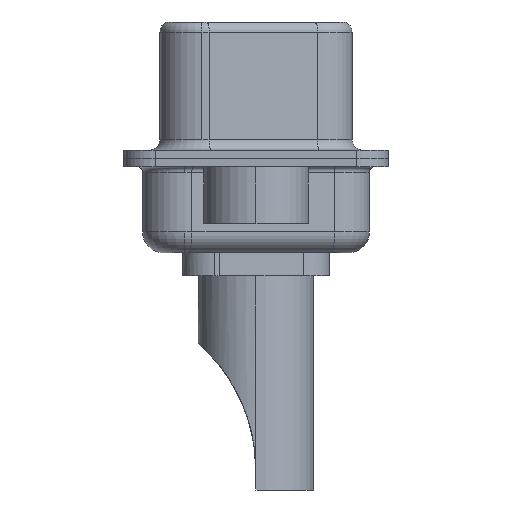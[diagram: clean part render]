
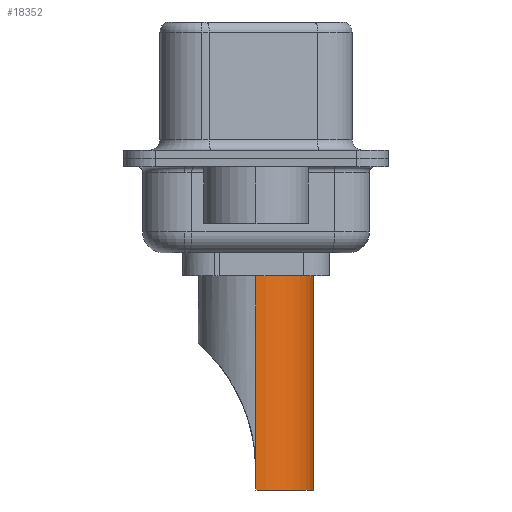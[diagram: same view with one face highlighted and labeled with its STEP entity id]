
A CAD part, left-side view. The second image highlights one B-rep face of the part: STEP entity #18352.
In plain terms, the highlighted cylindrical face has radius 2.75 mm (diameter 5.5 mm), a partial arc.
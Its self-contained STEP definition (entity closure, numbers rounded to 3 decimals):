
#19 = CARTESIAN_POINT ( 'NONE',  ( -2.75, 0., 4.234 ) ) ;
#313 = VECTOR ( 'NONE', #6127, 1000. ) ;
#859 = EDGE_CURVE ( 'NONE', #14765, #18203, #14205, .T. ) ;
#2672 = EDGE_LOOP ( 'NONE', ( #3869, #10466, #15259, #14167, #17523, #11882 ) ) ;
#2728 = CARTESIAN_POINT ( 'NONE',  ( -2.75, 0., -8.7 ) ) ;
#3127 = DIRECTION ( 'NONE',  ( 0., 0., 1. ) ) ;
#3869 = ORIENTED_EDGE ( 'NONE', *, *, #8987, .F. ) ;
#4400 = CIRCLE ( 'NONE', #14729, 2.75 ) ;
#5070 = AXIS2_PLACEMENT_3D ( 'NONE', #7988, #18836, #9633 ) ;
#5502 = VECTOR ( 'NONE', #15358, 1000. ) ;
#5547 = CARTESIAN_POINT ( 'NONE',  ( 2.75, 0., 1.5 ) ) ;
#5851 = CARTESIAN_POINT ( 'NONE',  ( 2.75, 0., 4.234 ) ) ;
#5928 = FACE_OUTER_BOUND ( 'NONE', #2672, .T. ) ;
#6127 = DIRECTION ( 'NONE',  ( 0., 0., -1. ) ) ;
#6656 = LINE ( 'NONE', #19, #15074 ) ;
#7647 = CARTESIAN_POINT ( 'NONE',  ( -2.75, 0., -8.7 ) ) ;
#7988 = CARTESIAN_POINT ( 'NONE',  ( 0., 0., -8.7 ) ) ;
#7994 = CARTESIAN_POINT ( 'NONE',  ( -2.75, 0., 1.5 ) ) ;
#8199 = LINE ( 'NONE', #7647, #313 ) ;
#8392 = DIRECTION ( 'NONE',  ( 0., 0., -1. ) ) ;
#8915 = EDGE_CURVE ( 'NONE', #16724, #17880, #8199, .T. ) ;
#8987 = EDGE_CURVE ( 'NONE', #16724, #19312, #6656, .T. ) ;
#9453 = VERTEX_POINT ( 'NONE', #5547 ) ;
#9493 = DIRECTION ( 'NONE',  ( 0., 0., 1. ) ) ;
#9633 = DIRECTION ( 'NONE',  ( 1., 0., 0. ) ) ;
#10131 = DIRECTION ( 'NONE',  ( 0., 0., 1. ) ) ;
#10466 = ORIENTED_EDGE ( 'NONE', *, *, #8915, .T. ) ;
#11324 = EDGE_CURVE ( 'NONE', #19312, #9453, #4400, .T. ) ;
#11882 = ORIENTED_EDGE ( 'NONE', *, *, #11324, .F. ) ;
#11993 = EDGE_CURVE ( 'NONE', #17880, #18203, #18045, .T. ) ;
#12673 = CARTESIAN_POINT ( 'NONE',  ( 0., 0., 1.5 ) ) ;
#13382 = CARTESIAN_POINT ( 'NONE',  ( 2.75, 0., -8.7 ) ) ;
#13949 = LINE ( 'NONE', #5851, #5502 ) ;
#14167 = ORIENTED_EDGE ( 'NONE', *, *, #859, .F. ) ;
#14188 = DIRECTION ( 'NONE',  ( 1., 0., 0. ) ) ;
#14205 = LINE ( 'NONE', #13382, #17719 ) ;
#14729 = AXIS2_PLACEMENT_3D ( 'NONE', #12673, #3127, #14188 ) ;
#14765 = VERTEX_POINT ( 'NONE', #15265 ) ;
#15074 = VECTOR ( 'NONE', #9493, 1000. ) ;
#15259 = ORIENTED_EDGE ( 'NONE', *, *, #11993, .T. ) ;
#15265 = CARTESIAN_POINT ( 'NONE',  ( 2.75, 0., -7.764 ) ) ;
#15358 = DIRECTION ( 'NONE',  ( 0., 0., 1. ) ) ;
#15800 = AXIS2_PLACEMENT_3D ( 'NONE', #16269, #10131, #19321 ) ;
#15940 = CARTESIAN_POINT ( 'NONE',  ( 2.75, 0., -8.7 ) ) ;
#16266 = EDGE_CURVE ( 'NONE', #14765, #9453, #13949, .T. ) ;
#16269 = CARTESIAN_POINT ( 'NONE',  ( 0., 0., 4.234 ) ) ;
#16724 = VERTEX_POINT ( 'NONE', #17004 ) ;
#17004 = CARTESIAN_POINT ( 'NONE',  ( -2.75, 0., -7.764 ) ) ;
#17377 = CYLINDRICAL_SURFACE ( 'NONE', #15800, 2.75 ) ;
#17523 = ORIENTED_EDGE ( 'NONE', *, *, #16266, .T. ) ;
#17719 = VECTOR ( 'NONE', #8392, 1000. ) ;
#17880 = VERTEX_POINT ( 'NONE', #2728 ) ;
#18045 = CIRCLE ( 'NONE', #5070, 2.75 ) ;
#18203 = VERTEX_POINT ( 'NONE', #15940 ) ;
#18352 = ADVANCED_FACE ( 'NONE', ( #5928 ), #17377, .T. ) ;
#18836 = DIRECTION ( 'NONE',  ( 0., 0., 1. ) ) ;
#19312 = VERTEX_POINT ( 'NONE', #7994 ) ;
#19321 = DIRECTION ( 'NONE',  ( 1., 0., 0. ) ) ;
